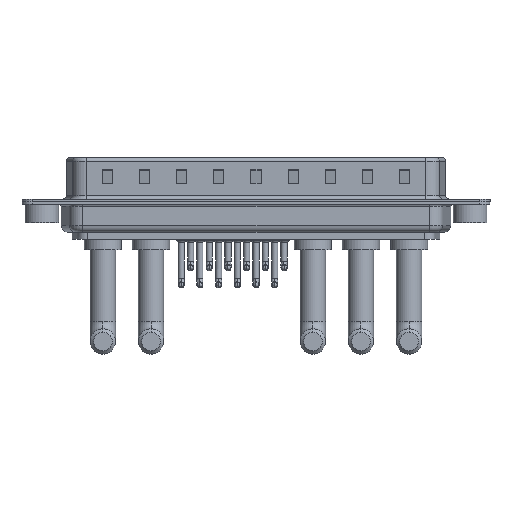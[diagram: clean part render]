
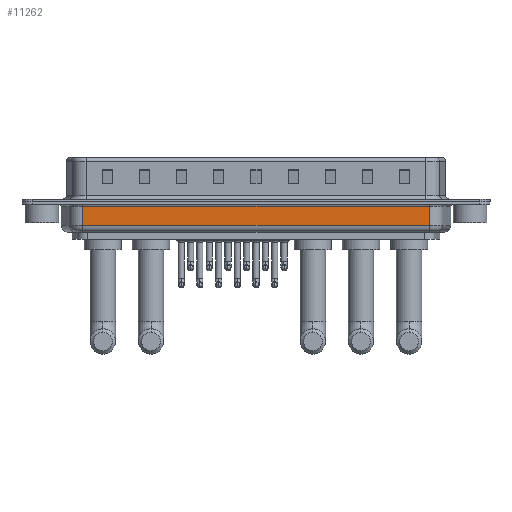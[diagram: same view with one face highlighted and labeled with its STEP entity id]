
A CAD part, front view. The second image highlights one B-rep face of the part: STEP entity #11262.
In plain terms, the highlighted planar face has unit normal (0, -1, 0).
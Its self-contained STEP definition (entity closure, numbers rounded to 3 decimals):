
#411 = ORIENTED_EDGE ( 'NONE', *, *, #16550, .T. ) ;
#912 = DIRECTION ( 'NONE',  ( 0., 1., 0. ) ) ;
#965 = VECTOR ( 'NONE', #2893, 1000. ) ;
#1039 = DIRECTION ( 'NONE',  ( -1., 0., 0. ) ) ;
#2195 = CARTESIAN_POINT ( 'NONE',  ( 6.031, -5.35, -3.5 ) ) ;
#2832 = LINE ( 'NONE', #8552, #23947 ) ;
#2893 = DIRECTION ( 'NONE',  ( 0., 0., 1. ) ) ;
#3163 = VERTEX_POINT ( 'NONE', #2195 ) ;
#4141 = AXIS2_PLACEMENT_3D ( 'NONE', #18716, #912, #1039 ) ;
#4574 = CARTESIAN_POINT ( 'NONE',  ( 57.469, -5.35, -4.5 ) ) ;
#4685 = VECTOR ( 'NONE', #18357, 1000. ) ;
#5757 = EDGE_LOOP ( 'NONE', ( #17706, #6759, #411, #13802 ) ) ;
#6604 = VERTEX_POINT ( 'NONE', #16989 ) ;
#6759 = ORIENTED_EDGE ( 'NONE', *, *, #24014, .T. ) ;
#7619 = CARTESIAN_POINT ( 'NONE',  ( 57.469, -5.35, -3.5 ) ) ;
#8234 = VECTOR ( 'NONE', #24266, 1000. ) ;
#8552 = CARTESIAN_POINT ( 'NONE',  ( 6.031, -5.35, -3.5 ) ) ;
#9731 = EDGE_CURVE ( 'NONE', #3163, #17714, #24146, .T. ) ;
#10438 = LINE ( 'NONE', #21859, #4685 ) ;
#10797 = PLANE ( 'NONE',  #4141 ) ;
#11262 = ADVANCED_FACE ( 'NONE', ( #18845 ), #10797, .F. ) ;
#12079 = CARTESIAN_POINT ( 'NONE',  ( 6.031, -5.35, -4.5 ) ) ;
#12829 = DIRECTION ( 'NONE',  ( 1., 0., 0. ) ) ;
#13802 = ORIENTED_EDGE ( 'NONE', *, *, #16463, .T. ) ;
#14318 = CARTESIAN_POINT ( 'NONE',  ( 6.031, -5.35, -0.65 ) ) ;
#14703 = LINE ( 'NONE', #4574, #965 ) ;
#16463 = EDGE_CURVE ( 'NONE', #6604, #17714, #10438, .T. ) ;
#16550 = EDGE_CURVE ( 'NONE', #17234, #6604, #14703, .T. ) ;
#16989 = CARTESIAN_POINT ( 'NONE',  ( 57.469, -5.35, -0.65 ) ) ;
#17234 = VERTEX_POINT ( 'NONE', #7619 ) ;
#17706 = ORIENTED_EDGE ( 'NONE', *, *, #9731, .F. ) ;
#17714 = VERTEX_POINT ( 'NONE', #14318 ) ;
#18357 = DIRECTION ( 'NONE',  ( -1., 0., 0. ) ) ;
#18716 = CARTESIAN_POINT ( 'NONE',  ( 6.031, -5.35, -4.5 ) ) ;
#18845 = FACE_OUTER_BOUND ( 'NONE', #5757, .T. ) ;
#21859 = CARTESIAN_POINT ( 'NONE',  ( 6.031, -5.35, -0.65 ) ) ;
#23947 = VECTOR ( 'NONE', #12829, 1000. ) ;
#24014 = EDGE_CURVE ( 'NONE', #3163, #17234, #2832, .T. ) ;
#24146 = LINE ( 'NONE', #12079, #8234 ) ;
#24266 = DIRECTION ( 'NONE',  ( 0., 0., 1. ) ) ;
